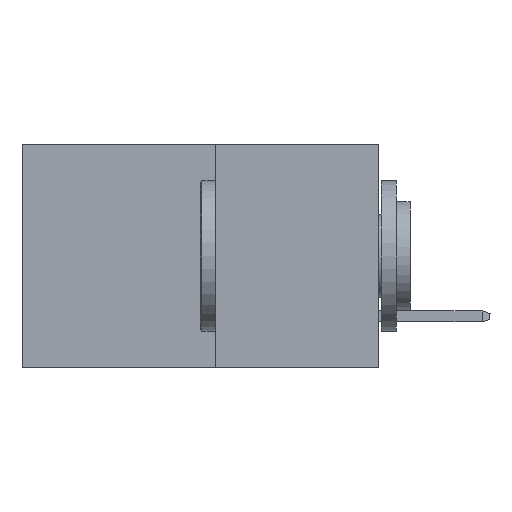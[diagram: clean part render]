
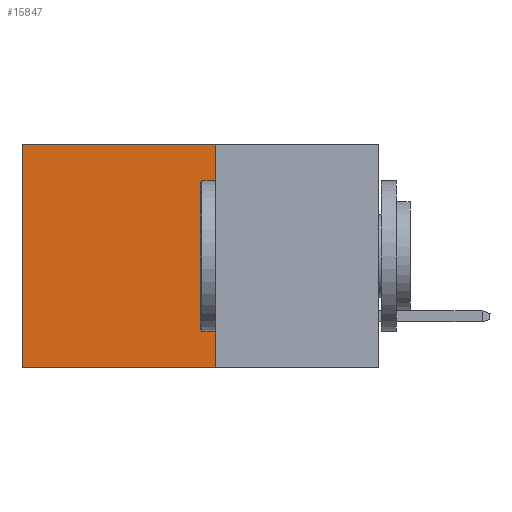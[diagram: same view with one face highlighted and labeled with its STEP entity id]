
A CAD part, left-side view. The second image highlights one B-rep face of the part: STEP entity #15847.
In plain terms, the highlighted planar face has unit normal (-1, 0, 0).
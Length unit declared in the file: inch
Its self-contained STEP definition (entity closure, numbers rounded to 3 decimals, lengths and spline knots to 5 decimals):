
#1497 = VERTEX_POINT ( 'NONE', #8945 ) ;
#2125 = LINE ( 'NONE', #15817, #12043 ) ;
#2765 = AXIS2_PLACEMENT_3D ( 'NONE', #13524, #14703, #7475 ) ;
#3347 = VERTEX_POINT ( 'NONE', #15132 ) ;
#3590 = LINE ( 'NONE', #13646, #7313 ) ;
#3919 = EDGE_LOOP ( 'NONE', ( #10295, #6338, #15681, #7086 ) ) ;
#4618 = LINE ( 'NONE', #5532, #13957 ) ;
#5022 = PLANE ( 'NONE',  #2765 ) ;
#5532 = CARTESIAN_POINT ( 'NONE',  ( 0.277, 0.59, -0.37 ) ) ;
#6037 = EDGE_CURVE ( 'NONE', #8527, #10155, #3590, .T. ) ;
#6291 = CARTESIAN_POINT ( 'NONE',  ( 0.277, 0.59, -0.37 ) ) ;
#6338 = ORIENTED_EDGE ( 'NONE', *, *, #6037, .F. ) ;
#6781 = DIRECTION ( 'NONE',  ( 0., 0., -1. ) ) ;
#7086 = ORIENTED_EDGE ( 'NONE', *, *, #13445, .T. ) ;
#7313 = VECTOR ( 'NONE', #13654, 39.37008 ) ;
#7475 = DIRECTION ( 'NONE',  ( 0., 0., -1. ) ) ;
#8142 = EDGE_CURVE ( 'NONE', #1497, #10155, #4618, .T. ) ;
#8527 = VERTEX_POINT ( 'NONE', #13357 ) ;
#8945 = CARTESIAN_POINT ( 'NONE',  ( 0.277, 0.59, 0. ) ) ;
#9433 = CARTESIAN_POINT ( 'NONE',  ( 0.277, 0.27, 0. ) ) ;
#9916 = DIRECTION ( 'NONE',  ( 0., 0., -1. ) ) ;
#10155 = VERTEX_POINT ( 'NONE', #6291 ) ;
#10295 = ORIENTED_EDGE ( 'NONE', *, *, #8142, .T. ) ;
#10636 = DIRECTION ( 'NONE',  ( 0., 1., 0. ) ) ;
#11475 = FACE_OUTER_BOUND ( 'NONE', #3919, .T. ) ;
#12043 = VECTOR ( 'NONE', #9916, 39.37008 ) ;
#12525 = LINE ( 'NONE', #9433, #14925 ) ;
#13357 = CARTESIAN_POINT ( 'NONE',  ( 0.277, 0.27, -0.37 ) ) ;
#13445 = EDGE_CURVE ( 'NONE', #3347, #1497, #12525, .T. ) ;
#13524 = CARTESIAN_POINT ( 'NONE',  ( 0.277, 0.27, -0.37 ) ) ;
#13646 = CARTESIAN_POINT ( 'NONE',  ( 0.277, 0.27, -0.37 ) ) ;
#13654 = DIRECTION ( 'NONE',  ( 0., 1., 0. ) ) ;
#13957 = VECTOR ( 'NONE', #6781, 39.37008 ) ;
#14703 = DIRECTION ( 'NONE',  ( 1., 0., 0. ) ) ;
#14925 = VECTOR ( 'NONE', #10636, 39.37008 ) ;
#15132 = CARTESIAN_POINT ( 'NONE',  ( 0.277, 0.27, 0. ) ) ;
#15596 = EDGE_CURVE ( 'NONE', #3347, #8527, #2125, .T. ) ;
#15681 = ORIENTED_EDGE ( 'NONE', *, *, #15596, .F. ) ;
#15817 = CARTESIAN_POINT ( 'NONE',  ( 0.277, 0.27, -0.37 ) ) ;
#15847 = ADVANCED_FACE ( 'NONE', ( #11475 ), #5022, .F. ) ;
